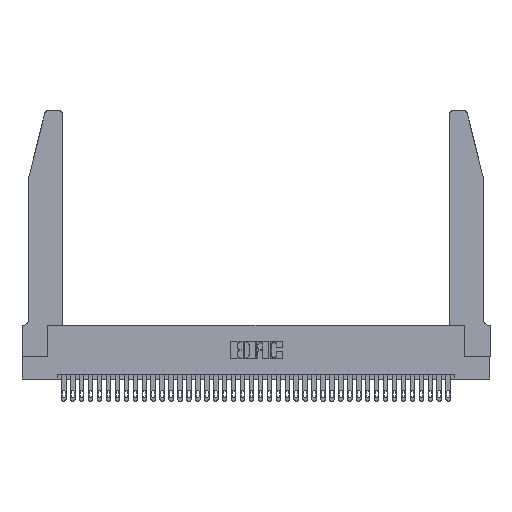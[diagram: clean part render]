
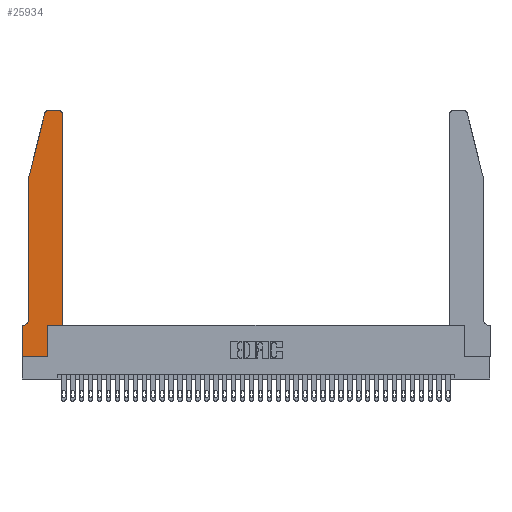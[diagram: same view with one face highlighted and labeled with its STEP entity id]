
A CAD part, top view. The second image highlights one B-rep face of the part: STEP entity #25934.
In plain terms, the highlighted planar face has unit normal (0, 0, 1).
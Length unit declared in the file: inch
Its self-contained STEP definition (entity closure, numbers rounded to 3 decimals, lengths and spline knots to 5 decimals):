
#356 = FACE_OUTER_BOUND ( 'NONE', #20591, .T. ) ;
#944 = ORIENTED_EDGE ( 'NONE', *, *, #25131, .T. ) ;
#1006 = CIRCLE ( 'NONE', #4369, 0.03 ) ;
#2153 = ORIENTED_EDGE ( 'NONE', *, *, #29005, .T. ) ;
#2830 = DIRECTION ( 'NONE',  ( 0., 0., 1. ) ) ;
#3259 = DIRECTION ( 'NONE',  ( 0., 1., 0. ) ) ;
#3497 = VECTOR ( 'NONE', #29763, 39.37008 ) ;
#3574 = VECTOR ( 'NONE', #13274, 39.37008 ) ;
#3847 = LINE ( 'NONE', #29076, #34936 ) ;
#4043 = AXIS2_PLACEMENT_3D ( 'NONE', #22108, #4303, #36942 ) ;
#4117 = LINE ( 'NONE', #26244, #29482 ) ;
#4303 = DIRECTION ( 'NONE',  ( 0., 0., -1. ) ) ;
#4369 = AXIS2_PLACEMENT_3D ( 'NONE', #20179, #23915, #26953 ) ;
#5132 = ORIENTED_EDGE ( 'NONE', *, *, #8459, .T. ) ;
#5264 = ORIENTED_EDGE ( 'NONE', *, *, #10027, .T. ) ;
#5377 = EDGE_CURVE ( 'NONE', #33721, #31046, #30962, .T. ) ;
#6098 = ORIENTED_EDGE ( 'NONE', *, *, #7615, .T. ) ;
#6461 = ORIENTED_EDGE ( 'NONE', *, *, #5377, .T. ) ;
#7231 = CIRCLE ( 'NONE', #23725, 0.03 ) ;
#7268 = CARTESIAN_POINT ( 'NONE',  ( 0.0755, 2., 0.37 ) ) ;
#7615 = EDGE_CURVE ( 'NONE', #21993, #33721, #35613, .T. ) ;
#8218 = LINE ( 'NONE', #32293, #17552 ) ;
#8459 = EDGE_CURVE ( 'NONE', #13356, #28712, #36917, .T. ) ;
#8518 = CARTESIAN_POINT ( 'NONE',  ( 0.0755, 2., 0.37 ) ) ;
#9136 = VECTOR ( 'NONE', #38959, 39.37008 ) ;
#9846 = LINE ( 'NONE', #10871, #29123 ) ;
#10027 = EDGE_CURVE ( 'NONE', #28712, #11560, #3847, .T. ) ;
#10871 = CARTESIAN_POINT ( 'NONE',  ( 0.2605, 2.75, 0.37 ) ) ;
#10987 = LINE ( 'NONE', #35484, #3497 ) ;
#11389 = DIRECTION ( 'NONE',  ( -1., 0., 0. ) ) ;
#11481 = VECTOR ( 'NONE', #3259, 39.37008 ) ;
#11516 = DIRECTION ( 'NONE',  ( 0., -1., 0. ) ) ;
#11560 = VERTEX_POINT ( 'NONE', #32645 ) ;
#12231 = EDGE_CURVE ( 'NONE', #11560, #34243, #1006, .T. ) ;
#12959 = CARTESIAN_POINT ( 'NONE',  ( 0.4505, 0.35, 0.37 ) ) ;
#13274 = DIRECTION ( 'NONE',  ( -0.239, -0.971, 0. ) ) ;
#13356 = VERTEX_POINT ( 'NONE', #14983 ) ;
#13411 = CARTESIAN_POINT ( 'NONE',  ( 0.284, 2.75, 0.37 ) ) ;
#13886 = DIRECTION ( 'NONE',  ( 0., -1., 0. ) ) ;
#14201 = CARTESIAN_POINT ( 'NONE',  ( 0., 0.35, 0.37 ) ) ;
#14718 = DIRECTION ( 'NONE',  ( 1., 0., 0. ) ) ;
#14983 = CARTESIAN_POINT ( 'NONE',  ( 0.2865, 0.35, 0.37 ) ) ;
#15817 = ORIENTED_EDGE ( 'NONE', *, *, #19044, .T. ) ;
#16974 = CIRCLE ( 'NONE', #4043, 0.07 ) ;
#17252 = DIRECTION ( 'NONE',  ( -1., 0., 0. ) ) ;
#17253 = CARTESIAN_POINT ( 'NONE',  ( 0.2865, 0.35, 0.37 ) ) ;
#17268 = ORIENTED_EDGE ( 'NONE', *, *, #24197, .T. ) ;
#17552 = VECTOR ( 'NONE', #11389, 39.37008 ) ;
#18315 = CARTESIAN_POINT ( 'NONE',  ( 0.25487, 2.72718, 0.37 ) ) ;
#19044 = EDGE_CURVE ( 'NONE', #32419, #25030, #4117, .T. ) ;
#20179 = CARTESIAN_POINT ( 'NONE',  ( 0.4205, 2.72, 0.37 ) ) ;
#20479 = DIRECTION ( 'NONE',  ( 0., 0., 1. ) ) ;
#20591 = EDGE_LOOP ( 'NONE', ( #944, #17268, #6098, #6461, #26758, #26583, #15817, #28818, #2153, #5132, #5264, #29346 ) ) ;
#20687 = AXIS2_PLACEMENT_3D ( 'NONE', #14201, #20479, #14718 ) ;
#20693 = CARTESIAN_POINT ( 'NONE',  ( 0.4505, 0.35, 0.37 ) ) ;
#20732 = CARTESIAN_POINT ( 'NONE',  ( 0.284, 2.72, 0.37 ) ) ;
#20969 = CARTESIAN_POINT ( 'NONE',  ( 0.0755, 0.42, 0.37 ) ) ;
#21993 = VERTEX_POINT ( 'NONE', #18315 ) ;
#22108 = CARTESIAN_POINT ( 'NONE',  ( 0.0055, 0.42, 0.37 ) ) ;
#22887 = VERTEX_POINT ( 'NONE', #34331 ) ;
#23725 = AXIS2_PLACEMENT_3D ( 'NONE', #20732, #2830, #36098 ) ;
#23915 = DIRECTION ( 'NONE',  ( 0., 0., 1. ) ) ;
#24043 = CARTESIAN_POINT ( 'NONE',  ( 0.0755, 2., 0.37 ) ) ;
#24197 = EDGE_CURVE ( 'NONE', #33463, #21993, #7231, .T. ) ;
#25030 = VERTEX_POINT ( 'NONE', #31637 ) ;
#25066 = VERTEX_POINT ( 'NONE', #34595 ) ;
#25131 = EDGE_CURVE ( 'NONE', #34243, #33463, #9846, .T. ) ;
#25934 = ADVANCED_FACE ( 'NONE', ( #356 ), #35456, .T. ) ;
#26244 = CARTESIAN_POINT ( 'NONE',  ( 0., 0., 0.37 ) ) ;
#26583 = ORIENTED_EDGE ( 'NONE', *, *, #28894, .T. ) ;
#26746 = VECTOR ( 'NONE', #11516, 39.37008 ) ;
#26758 = ORIENTED_EDGE ( 'NONE', *, *, #36483, .T. ) ;
#26953 = DIRECTION ( 'NONE',  ( 1., 0., 0. ) ) ;
#27429 = LINE ( 'NONE', #17253, #11481 ) ;
#28712 = VERTEX_POINT ( 'NONE', #12959 ) ;
#28818 = ORIENTED_EDGE ( 'NONE', *, *, #34978, .T. ) ;
#28894 = EDGE_CURVE ( 'NONE', #25066, #32419, #8218, .T. ) ;
#29005 = EDGE_CURVE ( 'NONE', #22887, #13356, #27429, .T. ) ;
#29076 = CARTESIAN_POINT ( 'NONE',  ( 0.4505, 0.35, 0.37 ) ) ;
#29123 = VECTOR ( 'NONE', #17252, 39.37008 ) ;
#29346 = ORIENTED_EDGE ( 'NONE', *, *, #12231, .T. ) ;
#29482 = VECTOR ( 'NONE', #13886, 39.37008 ) ;
#29763 = DIRECTION ( 'NONE',  ( 1., 0., 0. ) ) ;
#30962 = LINE ( 'NONE', #8518, #26746 ) ;
#31046 = VERTEX_POINT ( 'NONE', #20969 ) ;
#31637 = CARTESIAN_POINT ( 'NONE',  ( 0., 0., 0.37 ) ) ;
#32293 = CARTESIAN_POINT ( 'NONE',  ( 0.0755, 0.35, 0.37 ) ) ;
#32419 = VERTEX_POINT ( 'NONE', #36121 ) ;
#32595 = CARTESIAN_POINT ( 'NONE',  ( 0.4205, 2.75, 0.37 ) ) ;
#32645 = CARTESIAN_POINT ( 'NONE',  ( 0.4505, 2.72, 0.37 ) ) ;
#33463 = VERTEX_POINT ( 'NONE', #13411 ) ;
#33721 = VERTEX_POINT ( 'NONE', #24043 ) ;
#34243 = VERTEX_POINT ( 'NONE', #32595 ) ;
#34331 = CARTESIAN_POINT ( 'NONE',  ( 0.2865, 0., 0.37 ) ) ;
#34595 = CARTESIAN_POINT ( 'NONE',  ( 0.0055, 0.35, 0.37 ) ) ;
#34936 = VECTOR ( 'NONE', #37978, 39.37008 ) ;
#34978 = EDGE_CURVE ( 'NONE', #25030, #22887, #10987, .T. ) ;
#35456 = PLANE ( 'NONE',  #20687 ) ;
#35484 = CARTESIAN_POINT ( 'NONE',  ( 0., 0., 0.37 ) ) ;
#35613 = LINE ( 'NONE', #7268, #3574 ) ;
#36098 = DIRECTION ( 'NONE',  ( 1., 0., 0. ) ) ;
#36121 = CARTESIAN_POINT ( 'NONE',  ( 0., 0.35, 0.37 ) ) ;
#36483 = EDGE_CURVE ( 'NONE', #31046, #25066, #16974, .T. ) ;
#36917 = LINE ( 'NONE', #20693, #9136 ) ;
#36942 = DIRECTION ( 'NONE',  ( -1., 0., 0. ) ) ;
#37978 = DIRECTION ( 'NONE',  ( 0., 1., 0. ) ) ;
#38959 = DIRECTION ( 'NONE',  ( 1., 0., 0. ) ) ;
